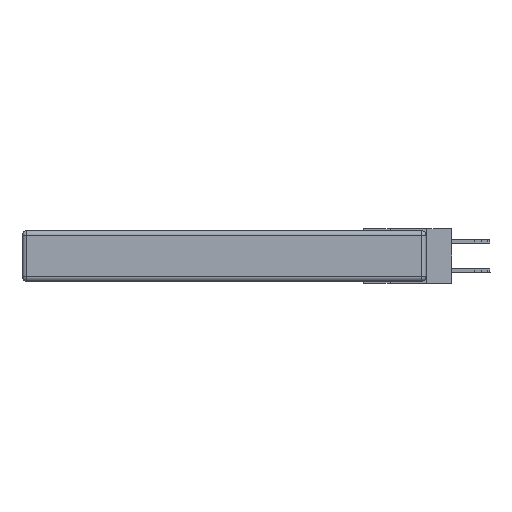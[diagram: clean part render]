
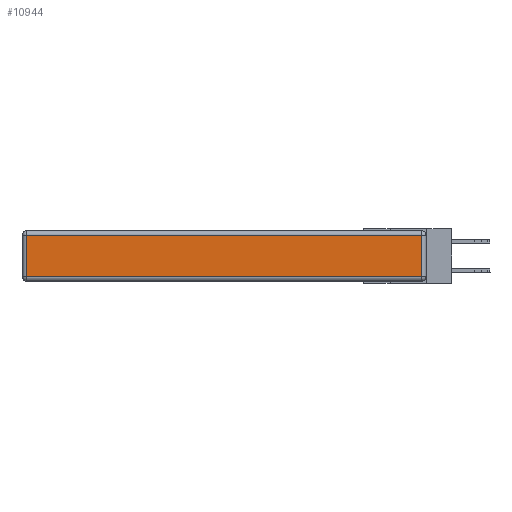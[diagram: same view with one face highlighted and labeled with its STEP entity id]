
A CAD part, left-side view. The second image highlights one B-rep face of the part: STEP entity #10944.
In plain terms, the highlighted planar face has unit normal (-1, 0, 0).
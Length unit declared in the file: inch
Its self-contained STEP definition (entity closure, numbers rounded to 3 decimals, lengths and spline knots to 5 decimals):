
#101 = DIRECTION ( 'NONE',  ( 0., 0., 1. ) ) ;
#1475 = VECTOR ( 'NONE', #101, 39.37008 ) ;
#2061 = VERTEX_POINT ( 'NONE', #2934 ) ;
#2529 = PLANE ( 'NONE',  #11353 ) ;
#2885 = DIRECTION ( 'NONE',  ( 0., 1., 0. ) ) ;
#2934 = CARTESIAN_POINT ( 'NONE',  ( 0., 0.03, -0.03 ) ) ;
#3418 = LINE ( 'NONE', #4128, #1475 ) ;
#3745 = DIRECTION ( 'NONE',  ( -1., 0., 0. ) ) ;
#4041 = CARTESIAN_POINT ( 'NONE',  ( 0., 2.75, -0.03 ) ) ;
#4128 = CARTESIAN_POINT ( 'NONE',  ( 0., 0.03, -0.343 ) ) ;
#4416 = EDGE_LOOP ( 'NONE', ( #6132, #14949, #7295, #16336 ) ) ;
#4551 = DIRECTION ( 'NONE',  ( 0., -1., 0. ) ) ;
#4918 = CARTESIAN_POINT ( 'NONE',  ( 0., 2.72, -0.343 ) ) ;
#4933 = VECTOR ( 'NONE', #2885, 39.37008 ) ;
#5284 = DIRECTION ( 'NONE',  ( 0., 0., 1. ) ) ;
#5646 = EDGE_CURVE ( 'NONE', #8803, #9029, #15441, .T. ) ;
#5980 = EDGE_CURVE ( 'NONE', #13206, #2061, #3418, .T. ) ;
#6132 = ORIENTED_EDGE ( 'NONE', *, *, #12888, .T. ) ;
#6483 = LINE ( 'NONE', #4041, #4933 ) ;
#7192 = VECTOR ( 'NONE', #4551, 39.37008 ) ;
#7295 = ORIENTED_EDGE ( 'NONE', *, *, #14110, .T. ) ;
#8025 = CARTESIAN_POINT ( 'NONE',  ( 0., 2.72, -0.313 ) ) ;
#8655 = CARTESIAN_POINT ( 'NONE',  ( 0., 2.72, -0.03 ) ) ;
#8701 = CARTESIAN_POINT ( 'NONE',  ( 0., 0., -0.313 ) ) ;
#8803 = VERTEX_POINT ( 'NONE', #8655 ) ;
#9029 = VERTEX_POINT ( 'NONE', #8025 ) ;
#10944 = ADVANCED_FACE ( 'NONE', ( #10960 ), #2529, .T. ) ;
#10960 = FACE_OUTER_BOUND ( 'NONE', #4416, .T. ) ;
#11023 = LINE ( 'NONE', #8701, #7192 ) ;
#11353 = AXIS2_PLACEMENT_3D ( 'NONE', #12290, #3745, #5284 ) ;
#12290 = CARTESIAN_POINT ( 'NONE',  ( 0., 0., -0.343 ) ) ;
#12305 = CARTESIAN_POINT ( 'NONE',  ( 0., 0.03, -0.313 ) ) ;
#12888 = EDGE_CURVE ( 'NONE', #9029, #13206, #11023, .T. ) ;
#13206 = VERTEX_POINT ( 'NONE', #12305 ) ;
#14110 = EDGE_CURVE ( 'NONE', #2061, #8803, #6483, .T. ) ;
#14332 = VECTOR ( 'NONE', #14603, 39.37008 ) ;
#14603 = DIRECTION ( 'NONE',  ( 0., 0., -1. ) ) ;
#14949 = ORIENTED_EDGE ( 'NONE', *, *, #5980, .T. ) ;
#15441 = LINE ( 'NONE', #4918, #14332 ) ;
#16336 = ORIENTED_EDGE ( 'NONE', *, *, #5646, .T. ) ;
